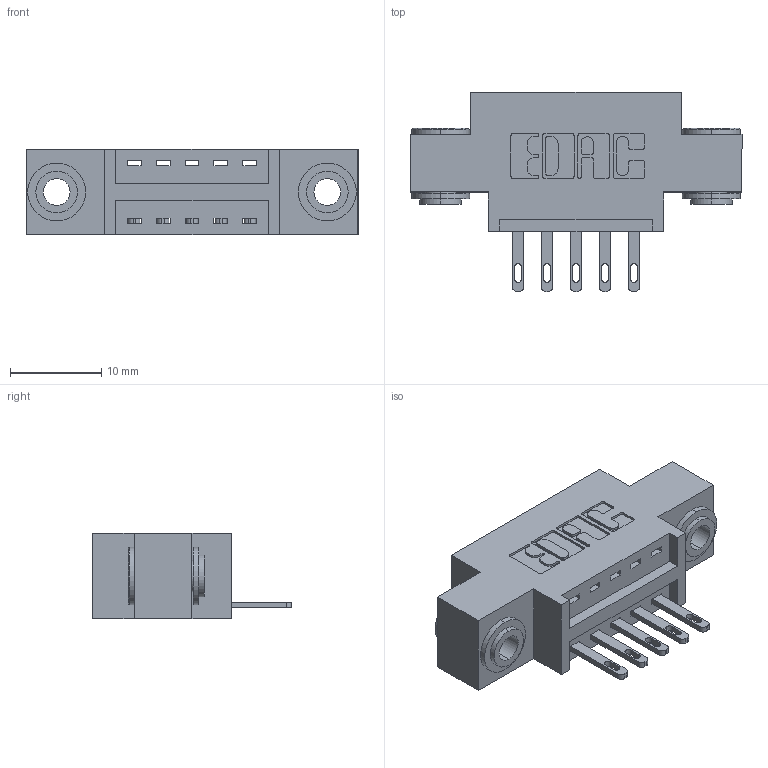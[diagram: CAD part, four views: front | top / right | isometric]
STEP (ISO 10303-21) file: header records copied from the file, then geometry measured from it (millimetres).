
FILE_DESCRIPTION (( 'STEP AP203' ), '1' );
FILE_NAME ('896-005-500-603.STEP', '2021-07-27T13:36:36', ( '' ), ( '' ), 'SwSTEP 2.0', 'SolidWorks 2020', '' );
FILE_SCHEMA (( 'CONFIG_CONTROL_DESIGN' ));
Length unit declared in the file: inch
Products named in the file (4): 345-292-001_345-293-100; 846 Part_0.170 Offset - 0.156 Dia-TH; 345-250-002_345-250-002-102; 896-005-500-603
Assembly tree (8 placements, depth 2):
  896-005-500-603
    846 Part_0.170 Offset - 0.156 Dia-TH
    345-292-001_345-293-100  x5
    345-250-002_345-250-002-102  x2
Bounding box: 36.45 x 21.84 x 9.4 mm (x, y, z)
Volume: 3101.9 mm3; surface area: 3868.9 mm2
Topology: 8 solids, 8 shells, 434 faces, 1257 edges, 834 vertices
Faces by surface type: plane 260, cylinder 166, cone 8
Entity records: 8796 total; most frequent: CARTESIAN_POINT 1498, ORIENTED_EDGE 1430, DIRECTION 1399, EDGE_CURVE 715, LINE 535, VECTOR 535, VERTEX_POINT 474, AXIS2_PLACEMENT_3D 432
